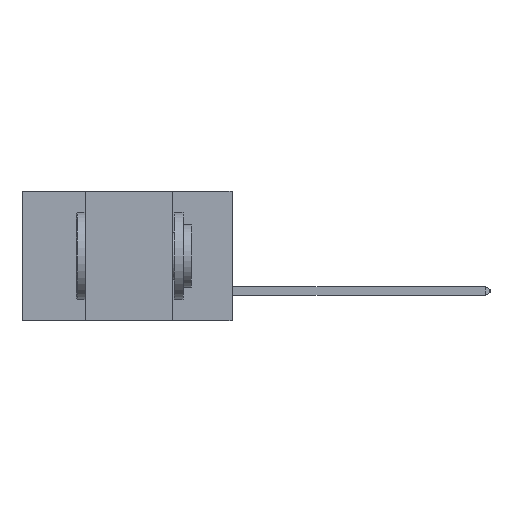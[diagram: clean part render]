
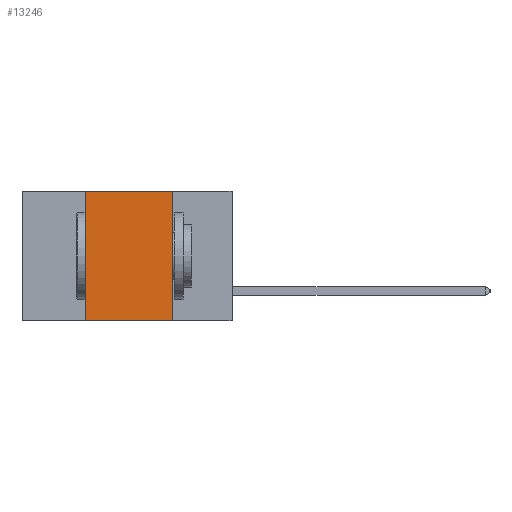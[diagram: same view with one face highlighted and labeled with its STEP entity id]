
A CAD part, left-side view. The second image highlights one B-rep face of the part: STEP entity #13246.
In plain terms, the highlighted planar face has unit normal (-1, 0, 0).
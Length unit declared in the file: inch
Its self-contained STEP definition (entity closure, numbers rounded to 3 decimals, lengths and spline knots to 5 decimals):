
#392 = VERTEX_POINT ( 'NONE', #20667 ) ;
#782 = VECTOR ( 'NONE', #19153, 39.37008 ) ;
#1243 = VERTEX_POINT ( 'NONE', #9881 ) ;
#1770 = ORIENTED_EDGE ( 'NONE', *, *, #16693, .T. ) ;
#1917 = EDGE_CURVE ( 'NONE', #392, #16141, #14268, .T. ) ;
#2881 = VECTOR ( 'NONE', #4714, 39.37008 ) ;
#4714 = DIRECTION ( 'NONE',  ( 0., 0., 1. ) ) ;
#4735 = DIRECTION ( 'NONE',  ( 0., -1., 0. ) ) ;
#5000 = CARTESIAN_POINT ( 'NONE',  ( 0., 0.42, -0.37 ) ) ;
#6101 = PLANE ( 'NONE',  #15678 ) ;
#6916 = DIRECTION ( 'NONE',  ( 0., -1., 0. ) ) ;
#6969 = LINE ( 'NONE', #10285, #11493 ) ;
#7226 = EDGE_LOOP ( 'NONE', ( #9551, #11660, #14660, #1770 ) ) ;
#7828 = DIRECTION ( 'NONE',  ( 1., 0., 0. ) ) ;
#9051 = LINE ( 'NONE', #14728, #13472 ) ;
#9551 = ORIENTED_EDGE ( 'NONE', *, *, #1917, .F. ) ;
#9881 = CARTESIAN_POINT ( 'NONE',  ( 0., 0.42, 0. ) ) ;
#10285 = CARTESIAN_POINT ( 'NONE',  ( 0., 0.6, -0.37 ) ) ;
#11331 = CARTESIAN_POINT ( 'NONE',  ( 0., 0.42, 0. ) ) ;
#11493 = VECTOR ( 'NONE', #6916, 39.37008 ) ;
#11660 = ORIENTED_EDGE ( 'NONE', *, *, #17765, .F. ) ;
#12853 = CARTESIAN_POINT ( 'NONE',  ( 0., 0.17, -0.37 ) ) ;
#12956 = VERTEX_POINT ( 'NONE', #5000 ) ;
#13031 = FACE_OUTER_BOUND ( 'NONE', #7226, .T. ) ;
#13246 = ADVANCED_FACE ( 'NONE', ( #13031 ), #6101, .F. ) ;
#13472 = VECTOR ( 'NONE', #4735, 39.37008 ) ;
#14268 = LINE ( 'NONE', #20329, #782 ) ;
#14660 = ORIENTED_EDGE ( 'NONE', *, *, #18246, .F. ) ;
#14728 = CARTESIAN_POINT ( 'NONE',  ( 0., 0.6, 0. ) ) ;
#15678 = AXIS2_PLACEMENT_3D ( 'NONE', #17560, #7828, #19083 ) ;
#16141 = VERTEX_POINT ( 'NONE', #12853 ) ;
#16179 = LINE ( 'NONE', #11331, #2881 ) ;
#16693 = EDGE_CURVE ( 'NONE', #12956, #16141, #6969, .T. ) ;
#17560 = CARTESIAN_POINT ( 'NONE',  ( 0., 0.6, 0. ) ) ;
#17765 = EDGE_CURVE ( 'NONE', #1243, #392, #9051, .T. ) ;
#18246 = EDGE_CURVE ( 'NONE', #12956, #1243, #16179, .T. ) ;
#19083 = DIRECTION ( 'NONE',  ( 0., 0., -1. ) ) ;
#19153 = DIRECTION ( 'NONE',  ( 0., 0., -1. ) ) ;
#20329 = CARTESIAN_POINT ( 'NONE',  ( 0., 0.17, 0. ) ) ;
#20667 = CARTESIAN_POINT ( 'NONE',  ( 0., 0.17, 0. ) ) ;
